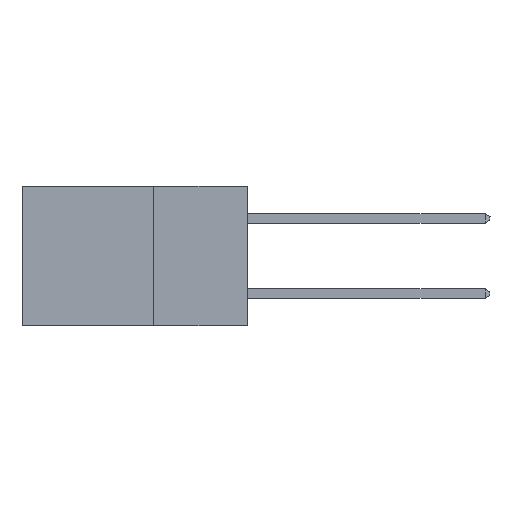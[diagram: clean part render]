
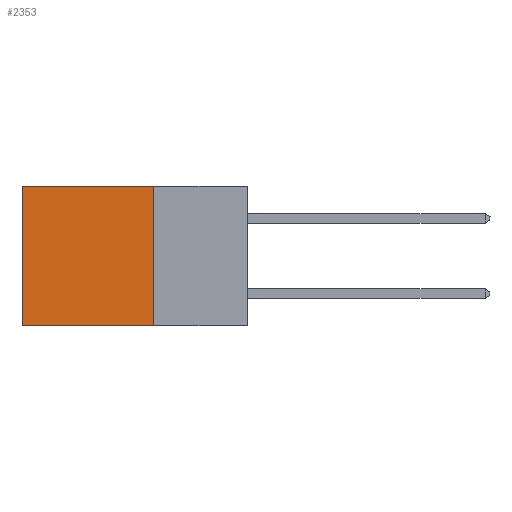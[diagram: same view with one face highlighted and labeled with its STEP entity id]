
A CAD part, left-side view. The second image highlights one B-rep face of the part: STEP entity #2353.
In plain terms, the highlighted planar face has unit normal (-1, 0, 0).
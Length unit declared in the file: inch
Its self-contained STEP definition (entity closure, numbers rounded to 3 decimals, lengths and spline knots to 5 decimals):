
#1131 = LINE ( 'NONE', #8527, #3213 ) ;
#2353 = ADVANCED_FACE ( 'NONE', ( #13326 ), #22332, .F. ) ;
#2379 = CARTESIAN_POINT ( 'NONE',  ( 0.2615, 0.25, -0.37 ) ) ;
#2734 = DIRECTION ( 'NONE',  ( 0., 0., -1. ) ) ;
#3117 = EDGE_CURVE ( 'NONE', #6293, #20352, #19967, .T. ) ;
#3128 = ORIENTED_EDGE ( 'NONE', *, *, #10950, .T. ) ;
#3213 = VECTOR ( 'NONE', #17675, 39.37008 ) ;
#3316 = CARTESIAN_POINT ( 'NONE',  ( 0.2615, 0.25, -0.37 ) ) ;
#3356 = CARTESIAN_POINT ( 'NONE',  ( 0.2615, 0.25, -0.37 ) ) ;
#4626 = CARTESIAN_POINT ( 'NONE',  ( 0.2615, 0.25, -0.37 ) ) ;
#6293 = VERTEX_POINT ( 'NONE', #13303 ) ;
#6387 = LINE ( 'NONE', #19392, #17762 ) ;
#7187 = VERTEX_POINT ( 'NONE', #8109 ) ;
#8109 = CARTESIAN_POINT ( 'NONE',  ( 0.2615, 0.6, 0. ) ) ;
#8527 = CARTESIAN_POINT ( 'NONE',  ( 0.2615, 0.25, 0. ) ) ;
#8974 = ORIENTED_EDGE ( 'NONE', *, *, #3117, .F. ) ;
#10738 = DIRECTION ( 'NONE',  ( 0., 0., -1. ) ) ;
#10749 = CARTESIAN_POINT ( 'NONE',  ( 0.2615, 0.6, -0.37 ) ) ;
#10950 = EDGE_CURVE ( 'NONE', #6293, #7187, #1131, .T. ) ;
#12205 = ORIENTED_EDGE ( 'NONE', *, *, #15873, .F. ) ;
#12979 = DIRECTION ( 'NONE',  ( 1., 0., 0. ) ) ;
#13303 = CARTESIAN_POINT ( 'NONE',  ( 0.2615, 0.25, 0. ) ) ;
#13326 = FACE_OUTER_BOUND ( 'NONE', #18876, .T. ) ;
#15015 = LINE ( 'NONE', #3356, #20763 ) ;
#15119 = ORIENTED_EDGE ( 'NONE', *, *, #18244, .T. ) ;
#15873 = EDGE_CURVE ( 'NONE', #20352, #19713, #15015, .T. ) ;
#17675 = DIRECTION ( 'NONE',  ( 0., 1., 0. ) ) ;
#17762 = VECTOR ( 'NONE', #2734, 39.37008 ) ;
#18244 = EDGE_CURVE ( 'NONE', #7187, #19713, #6387, .T. ) ;
#18801 = DIRECTION ( 'NONE',  ( 0., 0., -1. ) ) ;
#18876 = EDGE_LOOP ( 'NONE', ( #15119, #12205, #8974, #3128 ) ) ;
#19292 = VECTOR ( 'NONE', #10738, 39.37008 ) ;
#19392 = CARTESIAN_POINT ( 'NONE',  ( 0.2615, 0.6, -0.37 ) ) ;
#19713 = VERTEX_POINT ( 'NONE', #10749 ) ;
#19967 = LINE ( 'NONE', #3316, #19292 ) ;
#20352 = VERTEX_POINT ( 'NONE', #4626 ) ;
#20606 = DIRECTION ( 'NONE',  ( 0., 1., 0. ) ) ;
#20763 = VECTOR ( 'NONE', #20606, 39.37008 ) ;
#21833 = AXIS2_PLACEMENT_3D ( 'NONE', #2379, #12979, #18801 ) ;
#22332 = PLANE ( 'NONE',  #21833 ) ;
